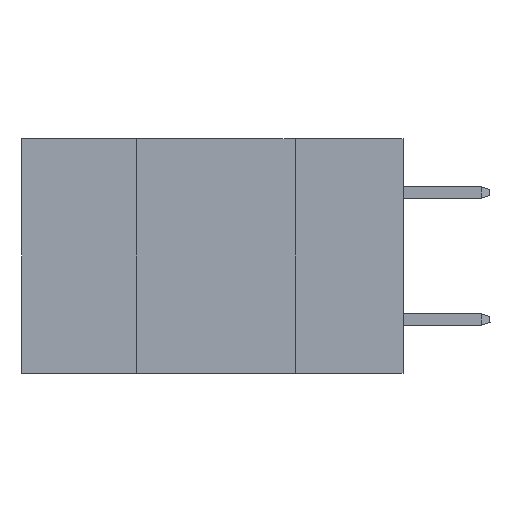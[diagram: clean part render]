
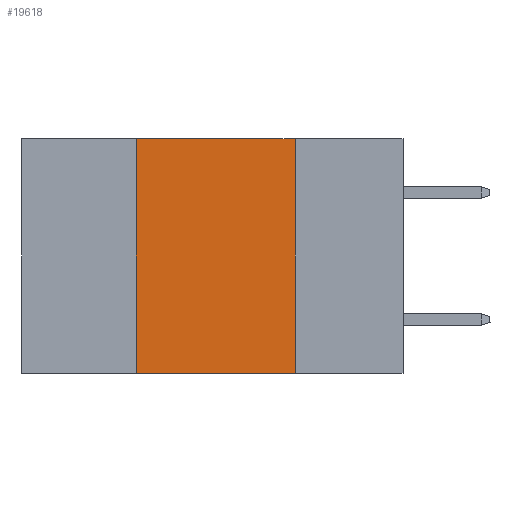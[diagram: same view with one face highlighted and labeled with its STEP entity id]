
A CAD part, left-side view. The second image highlights one B-rep face of the part: STEP entity #19618.
In plain terms, the highlighted planar face has unit normal (-1, 0, 0).
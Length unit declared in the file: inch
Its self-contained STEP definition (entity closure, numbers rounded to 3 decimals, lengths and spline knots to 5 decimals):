
#9 = EDGE_CURVE ( 'NONE', #20770, #6534, #23767, .T. ) ;
#656 = VECTOR ( 'NONE', #9007, 39.37008 ) ;
#1166 = CARTESIAN_POINT ( 'NONE',  ( 0., 0.42, 0. ) ) ;
#1254 = VECTOR ( 'NONE', #19695, 39.37008 ) ;
#1455 = DIRECTION ( 'NONE',  ( 0., -1., 0. ) ) ;
#1869 = ORIENTED_EDGE ( 'NONE', *, *, #23717, .F. ) ;
#2352 = ORIENTED_EDGE ( 'NONE', *, *, #10606, .T. ) ;
#2424 = VECTOR ( 'NONE', #6865, 39.37008 ) ;
#2655 = ORIENTED_EDGE ( 'NONE', *, *, #10227, .F. ) ;
#3679 = DIRECTION ( 'NONE',  ( 0., 0., -1. ) ) ;
#4044 = EDGE_LOOP ( 'NONE', ( #17559, #1869, #2655, #2352 ) ) ;
#5238 = CARTESIAN_POINT ( 'NONE',  ( 0., 0.42, 0. ) ) ;
#6145 = CARTESIAN_POINT ( 'NONE',  ( 0., 0.42, -0.37 ) ) ;
#6534 = VERTEX_POINT ( 'NONE', #6680 ) ;
#6680 = CARTESIAN_POINT ( 'NONE',  ( 0., 0.17, -0.37 ) ) ;
#6823 = CARTESIAN_POINT ( 'NONE',  ( 0., 0.6, 0. ) ) ;
#6865 = DIRECTION ( 'NONE',  ( 0., -1., 0. ) ) ;
#7696 = PLANE ( 'NONE',  #15298 ) ;
#9007 = DIRECTION ( 'NONE',  ( 0., 0., -1. ) ) ;
#10227 = EDGE_CURVE ( 'NONE', #23096, #19859, #15937, .T. ) ;
#10604 = LINE ( 'NONE', #6823, #13168 ) ;
#10606 = EDGE_CURVE ( 'NONE', #23096, #6534, #18440, .T. ) ;
#10749 = CARTESIAN_POINT ( 'NONE',  ( 0., 0.17, 0. ) ) ;
#10828 = CARTESIAN_POINT ( 'NONE',  ( 0., 0.17, 0. ) ) ;
#11098 = DIRECTION ( 'NONE',  ( 1., 0., 0. ) ) ;
#11589 = FACE_OUTER_BOUND ( 'NONE', #4044, .T. ) ;
#13168 = VECTOR ( 'NONE', #1455, 39.37008 ) ;
#15298 = AXIS2_PLACEMENT_3D ( 'NONE', #20358, #11098, #3679 ) ;
#15937 = LINE ( 'NONE', #1166, #1254 ) ;
#17559 = ORIENTED_EDGE ( 'NONE', *, *, #9, .F. ) ;
#18440 = LINE ( 'NONE', #24061, #2424 ) ;
#19618 = ADVANCED_FACE ( 'NONE', ( #11589 ), #7696, .F. ) ;
#19695 = DIRECTION ( 'NONE',  ( 0., 0., 1. ) ) ;
#19859 = VERTEX_POINT ( 'NONE', #5238 ) ;
#20358 = CARTESIAN_POINT ( 'NONE',  ( 0., 0.6, 0. ) ) ;
#20770 = VERTEX_POINT ( 'NONE', #10749 ) ;
#23096 = VERTEX_POINT ( 'NONE', #6145 ) ;
#23717 = EDGE_CURVE ( 'NONE', #19859, #20770, #10604, .T. ) ;
#23767 = LINE ( 'NONE', #10828, #656 ) ;
#24061 = CARTESIAN_POINT ( 'NONE',  ( 0., 0.6, -0.37 ) ) ;
